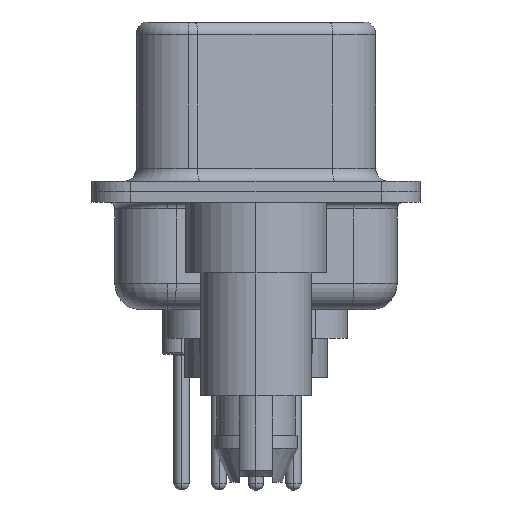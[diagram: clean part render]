
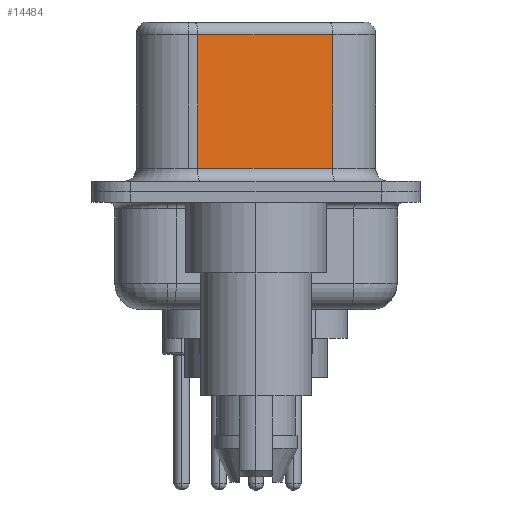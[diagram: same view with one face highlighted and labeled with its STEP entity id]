
A CAD part, left-side view. The second image highlights one B-rep face of the part: STEP entity #14484.
In plain terms, the highlighted planar face has unit normal (-0.985, -0.174, 0).
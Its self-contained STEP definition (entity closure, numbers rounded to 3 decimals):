
#478 = ORIENTED_EDGE ( 'NONE', *, *, #18679, .T. ) ;
#1609 = VERTEX_POINT ( 'NONE', #6271 ) ;
#2755 = EDGE_CURVE ( 'NONE', #16892, #5545, #20666, .T. ) ;
#2897 = DIRECTION ( 'NONE',  ( 0., 0., -1. ) ) ;
#2913 = CARTESIAN_POINT ( 'NONE',  ( 4.585, -2.927, 6.02 ) ) ;
#4701 = CARTESIAN_POINT ( 'NONE',  ( 3.675, 2.233, 0.9 ) ) ;
#5413 = VECTOR ( 'NONE', #11111, 1000. ) ;
#5545 = VERTEX_POINT ( 'NONE', #6118 ) ;
#6118 = CARTESIAN_POINT ( 'NONE',  ( 4.585, -2.927, 0.9 ) ) ;
#6271 = CARTESIAN_POINT ( 'NONE',  ( 3.675, 2.233, 6.02 ) ) ;
#6924 = PLANE ( 'NONE',  #12850 ) ;
#8616 = DIRECTION ( 'NONE',  ( 0., 0., -1. ) ) ;
#8950 = LINE ( 'NONE', #17560, #18132 ) ;
#10049 = DIRECTION ( 'NONE',  ( -0.174, 0.985, 0. ) ) ;
#11111 = DIRECTION ( 'NONE',  ( -0.174, 0.985, 0. ) ) ;
#11120 = LINE ( 'NONE', #2913, #5413 ) ;
#11161 = LINE ( 'NONE', #16933, #21107 ) ;
#11799 = VECTOR ( 'NONE', #18110, 1000. ) ;
#12608 = CARTESIAN_POINT ( 'NONE',  ( 4.585, -2.927, 0.9 ) ) ;
#12820 = EDGE_CURVE ( 'NONE', #1609, #16892, #11161, .T. ) ;
#12850 = AXIS2_PLACEMENT_3D ( 'NONE', #13634, #20346, #10049 ) ;
#13634 = CARTESIAN_POINT ( 'NONE',  ( 4.585, -2.927, 6.52 ) ) ;
#14081 = CARTESIAN_POINT ( 'NONE',  ( 4.585, -2.927, 6.02 ) ) ;
#14484 = ADVANCED_FACE ( 'NONE', ( #14810 ), #6924, .F. ) ;
#14810 = FACE_OUTER_BOUND ( 'NONE', #19631, .T. ) ;
#15822 = VERTEX_POINT ( 'NONE', #14081 ) ;
#16892 = VERTEX_POINT ( 'NONE', #4701 ) ;
#16933 = CARTESIAN_POINT ( 'NONE',  ( 3.675, 2.233, 6.52 ) ) ;
#17560 = CARTESIAN_POINT ( 'NONE',  ( 4.585, -2.927, 6.52 ) ) ;
#18110 = DIRECTION ( 'NONE',  ( 0.174, -0.985, 0. ) ) ;
#18132 = VECTOR ( 'NONE', #2897, 1000. ) ;
#18556 = ORIENTED_EDGE ( 'NONE', *, *, #2755, .T. ) ;
#18677 = ORIENTED_EDGE ( 'NONE', *, *, #12820, .T. ) ;
#18679 = EDGE_CURVE ( 'NONE', #15822, #1609, #11120, .T. ) ;
#19631 = EDGE_LOOP ( 'NONE', ( #20791, #478, #18677, #18556 ) ) ;
#20346 = DIRECTION ( 'NONE',  ( 0.985, 0.174, 0. ) ) ;
#20666 = LINE ( 'NONE', #12608, #11799 ) ;
#20791 = ORIENTED_EDGE ( 'NONE', *, *, #21178, .F. ) ;
#21107 = VECTOR ( 'NONE', #8616, 1000. ) ;
#21178 = EDGE_CURVE ( 'NONE', #15822, #5545, #8950, .T. ) ;
